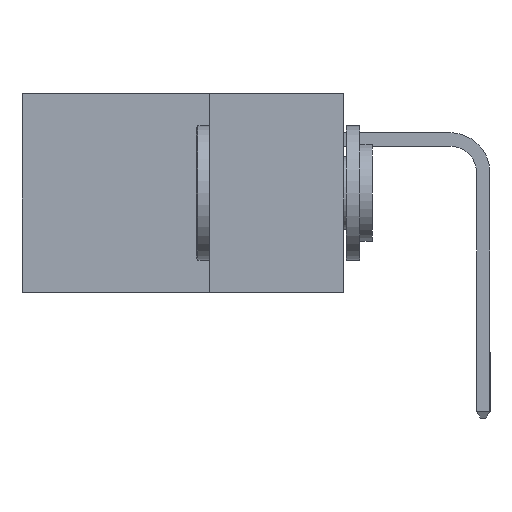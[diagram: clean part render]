
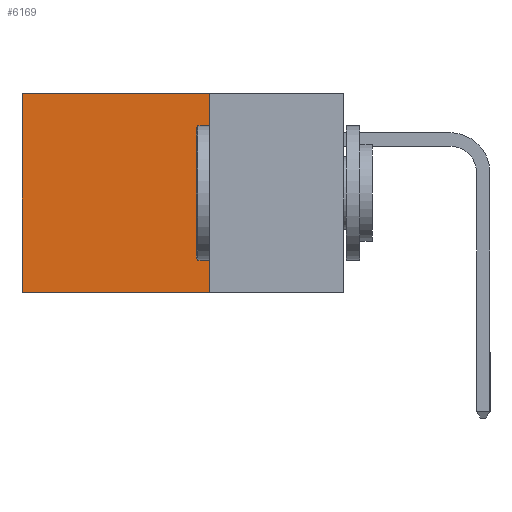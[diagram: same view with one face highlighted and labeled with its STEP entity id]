
A CAD part, left-side view. The second image highlights one B-rep face of the part: STEP entity #6169.
In plain terms, the highlighted planar face has unit normal (-1, 0, 0).
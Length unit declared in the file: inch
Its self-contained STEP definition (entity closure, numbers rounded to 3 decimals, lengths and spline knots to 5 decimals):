
#896 = VERTEX_POINT ( 'NONE', #17512 ) ;
#1074 = CARTESIAN_POINT ( 'NONE',  ( 0.298, 0.25, 0. ) ) ;
#1669 = CARTESIAN_POINT ( 'NONE',  ( 0.298, 0.6, 0. ) ) ;
#1776 = VERTEX_POINT ( 'NONE', #16794 ) ;
#3560 = ORIENTED_EDGE ( 'NONE', *, *, #18096, .F. ) ;
#3645 = VECTOR ( 'NONE', #5019, 39.37008 ) ;
#3718 = ORIENTED_EDGE ( 'NONE', *, *, #17755, .T. ) ;
#5019 = DIRECTION ( 'NONE',  ( 0., 0., -1. ) ) ;
#6070 = CARTESIAN_POINT ( 'NONE',  ( 0.298, 0.25, -0.37 ) ) ;
#6104 = CARTESIAN_POINT ( 'NONE',  ( 0.298, 0.6, 0. ) ) ;
#6169 = ADVANCED_FACE ( 'NONE', ( #12054 ), #12636, .F. ) ;
#6540 = CARTESIAN_POINT ( 'NONE',  ( 0.298, 0.25, 0. ) ) ;
#6587 = DIRECTION ( 'NONE',  ( 0., 0., -1. ) ) ;
#6748 = DIRECTION ( 'NONE',  ( 0., 1., 0. ) ) ;
#6834 = LINE ( 'NONE', #1669, #3645 ) ;
#7359 = VECTOR ( 'NONE', #10479, 39.37008 ) ;
#7603 = LINE ( 'NONE', #9822, #15870 ) ;
#7656 = DIRECTION ( 'NONE',  ( 0., 1., 0. ) ) ;
#9439 = VECTOR ( 'NONE', #7656, 39.37008 ) ;
#9822 = CARTESIAN_POINT ( 'NONE',  ( 0.298, 0.25, 0. ) ) ;
#10479 = DIRECTION ( 'NONE',  ( 0., 0., -1. ) ) ;
#12054 = FACE_OUTER_BOUND ( 'NONE', #12622, .T. ) ;
#12622 = EDGE_LOOP ( 'NONE', ( #15982, #18702, #3560, #3718 ) ) ;
#12636 = PLANE ( 'NONE',  #15621 ) ;
#12767 = DIRECTION ( 'NONE',  ( 1., 0., 0. ) ) ;
#14227 = CARTESIAN_POINT ( 'NONE',  ( 0.298, 0.25, 0. ) ) ;
#14627 = VERTEX_POINT ( 'NONE', #6540 ) ;
#15621 = AXIS2_PLACEMENT_3D ( 'NONE', #14227, #12767, #6587 ) ;
#15870 = VECTOR ( 'NONE', #6748, 39.37008 ) ;
#15982 = ORIENTED_EDGE ( 'NONE', *, *, #18416, .T. ) ;
#16794 = CARTESIAN_POINT ( 'NONE',  ( 0.298, 0.25, -0.37 ) ) ;
#16971 = VERTEX_POINT ( 'NONE', #6104 ) ;
#17512 = CARTESIAN_POINT ( 'NONE',  ( 0.298, 0.6, -0.37 ) ) ;
#17587 = LINE ( 'NONE', #1074, #7359 ) ;
#17755 = EDGE_CURVE ( 'NONE', #14627, #16971, #7603, .T. ) ;
#18096 = EDGE_CURVE ( 'NONE', #14627, #1776, #17587, .T. ) ;
#18416 = EDGE_CURVE ( 'NONE', #16971, #896, #6834, .T. ) ;
#18702 = ORIENTED_EDGE ( 'NONE', *, *, #18975, .F. ) ;
#18975 = EDGE_CURVE ( 'NONE', #1776, #896, #20054, .T. ) ;
#20054 = LINE ( 'NONE', #6070, #9439 ) ;
